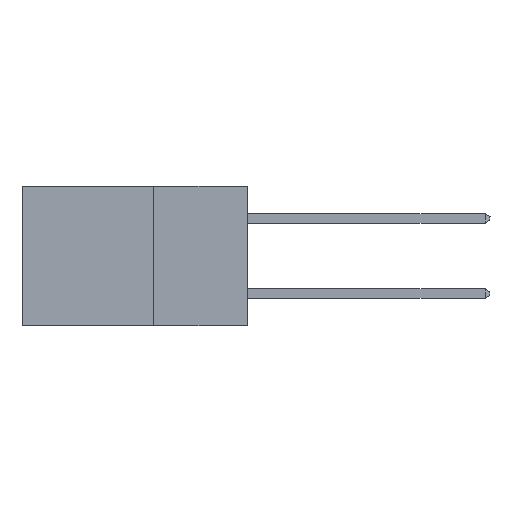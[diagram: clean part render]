
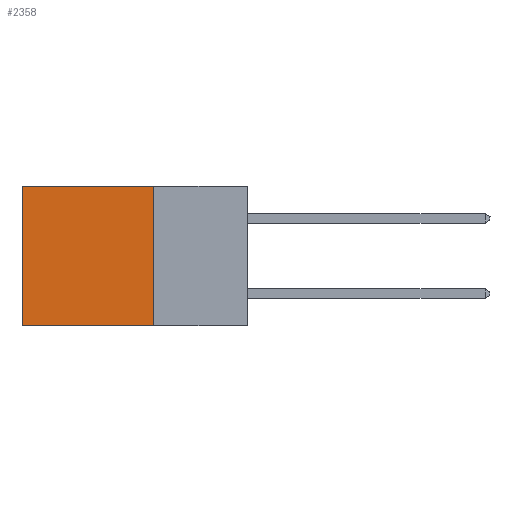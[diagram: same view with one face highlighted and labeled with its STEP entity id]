
A CAD part, left-side view. The second image highlights one B-rep face of the part: STEP entity #2358.
In plain terms, the highlighted planar face has unit normal (-1, 0, 0).
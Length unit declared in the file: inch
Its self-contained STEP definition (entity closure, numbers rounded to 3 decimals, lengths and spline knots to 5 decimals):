
#135 = EDGE_LOOP ( 'NONE', ( #1813, #28873, #19023, #10800 ) ) ;
#1813 = ORIENTED_EDGE ( 'NONE', *, *, #29493, .T. ) ;
#2358 = ADVANCED_FACE ( 'NONE', ( #20129 ), #22639, .F. ) ;
#3847 = VERTEX_POINT ( 'NONE', #17254 ) ;
#4161 = VECTOR ( 'NONE', #17973, 39.37008 ) ;
#5333 = CARTESIAN_POINT ( 'NONE',  ( 0.298, 0.6, -0.37 ) ) ;
#9381 = LINE ( 'NONE', #15642, #14634 ) ;
#9500 = VERTEX_POINT ( 'NONE', #28660 ) ;
#10800 = ORIENTED_EDGE ( 'NONE', *, *, #14382, .T. ) ;
#12625 = EDGE_CURVE ( 'NONE', #3847, #9500, #32276, .T. ) ;
#12754 = AXIS2_PLACEMENT_3D ( 'NONE', #28581, #29735, #25229 ) ;
#13206 = VERTEX_POINT ( 'NONE', #25304 ) ;
#14158 = VECTOR ( 'NONE', #17031, 39.37008 ) ;
#14382 = EDGE_CURVE ( 'NONE', #3847, #13206, #17749, .T. ) ;
#14634 = VECTOR ( 'NONE', #28372, 39.37008 ) ;
#14949 = LINE ( 'NONE', #27175, #14158 ) ;
#15222 = VERTEX_POINT ( 'NONE', #5333 ) ;
#15642 = CARTESIAN_POINT ( 'NONE',  ( 0.298, 0.6, 0. ) ) ;
#17031 = DIRECTION ( 'NONE',  ( 0., 1., 0. ) ) ;
#17254 = CARTESIAN_POINT ( 'NONE',  ( 0.298, 0.25, 0. ) ) ;
#17749 = LINE ( 'NONE', #19422, #23731 ) ;
#17973 = DIRECTION ( 'NONE',  ( 0., 0., -1. ) ) ;
#19023 = ORIENTED_EDGE ( 'NONE', *, *, #12625, .F. ) ;
#19422 = CARTESIAN_POINT ( 'NONE',  ( 0.298, 0.25, 0. ) ) ;
#20129 = FACE_OUTER_BOUND ( 'NONE', #135, .T. ) ;
#22639 = PLANE ( 'NONE',  #12754 ) ;
#23731 = VECTOR ( 'NONE', #24546, 39.37008 ) ;
#24546 = DIRECTION ( 'NONE',  ( 0., 1., 0. ) ) ;
#25229 = DIRECTION ( 'NONE',  ( 0., 0., -1. ) ) ;
#25304 = CARTESIAN_POINT ( 'NONE',  ( 0.298, 0.6, 0. ) ) ;
#25785 = CARTESIAN_POINT ( 'NONE',  ( 0.298, 0.25, 0. ) ) ;
#27175 = CARTESIAN_POINT ( 'NONE',  ( 0.298, 0.25, -0.37 ) ) ;
#28372 = DIRECTION ( 'NONE',  ( 0., 0., -1. ) ) ;
#28581 = CARTESIAN_POINT ( 'NONE',  ( 0.298, 0.25, 0. ) ) ;
#28660 = CARTESIAN_POINT ( 'NONE',  ( 0.298, 0.25, -0.37 ) ) ;
#28873 = ORIENTED_EDGE ( 'NONE', *, *, #30585, .F. ) ;
#29493 = EDGE_CURVE ( 'NONE', #13206, #15222, #9381, .T. ) ;
#29735 = DIRECTION ( 'NONE',  ( 1., 0., 0. ) ) ;
#30585 = EDGE_CURVE ( 'NONE', #9500, #15222, #14949, .T. ) ;
#32276 = LINE ( 'NONE', #25785, #4161 ) ;
